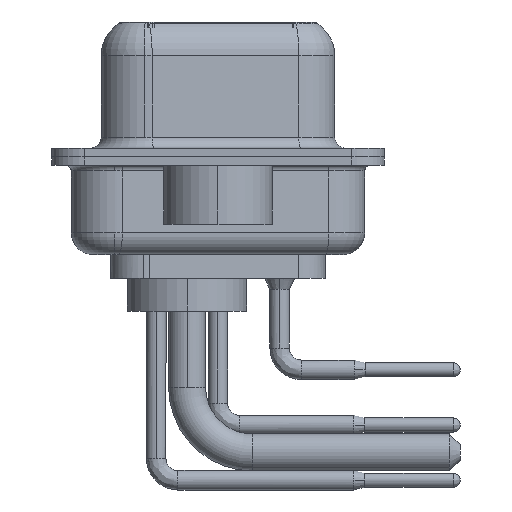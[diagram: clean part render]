
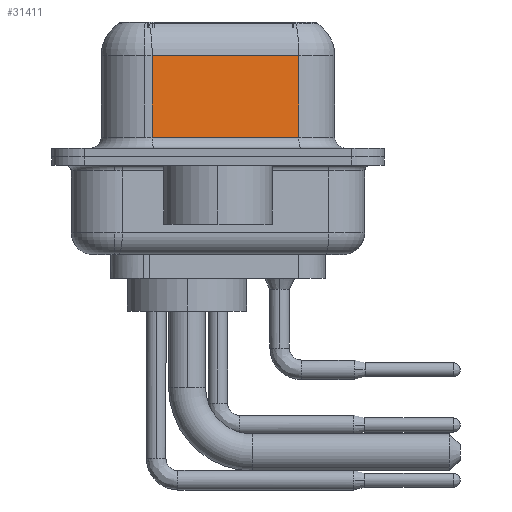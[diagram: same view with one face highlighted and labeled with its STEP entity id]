
A CAD part, left-side view. The second image highlights one B-rep face of the part: STEP entity #31411.
In plain terms, the highlighted planar face has unit normal (-0.985, -0.174, 0).
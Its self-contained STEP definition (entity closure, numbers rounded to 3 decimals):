
#448 = DIRECTION ( 'NONE',  ( 0.174, -0.985, 0. ) ) ;
#1544 = PLANE ( 'NONE',  #31819 ) ;
#2123 = EDGE_LOOP ( 'NONE', ( #21889, #3475, #9913, #14972 ) ) ;
#2804 = LINE ( 'NONE', #12839, #31920 ) ;
#3475 = ORIENTED_EDGE ( 'NONE', *, *, #16278, .T. ) ;
#3918 = DIRECTION ( 'NONE',  ( -0.174, 0.985, 0. ) ) ;
#3994 = EDGE_CURVE ( 'NONE', #17035, #30878, #7705, .T. ) ;
#4028 = DIRECTION ( 'NONE',  ( 0.985, 0.174, 0. ) ) ;
#5086 = CARTESIAN_POINT ( 'NONE',  ( 5.621, -3.722, 6.4 ) ) ;
#5248 = EDGE_CURVE ( 'NONE', #15161, #30878, #13133, .T. ) ;
#6377 = CARTESIAN_POINT ( 'NONE',  ( 5.621, -3.722, 0.9 ) ) ;
#7705 = LINE ( 'NONE', #5086, #16995 ) ;
#9243 = VECTOR ( 'NONE', #3918, 1000. ) ;
#9913 = ORIENTED_EDGE ( 'NONE', *, *, #10064, .T. ) ;
#10064 = EDGE_CURVE ( 'NONE', #23374, #15161, #2804, .T. ) ;
#10382 = DIRECTION ( 'NONE',  ( 0., 0., -1. ) ) ;
#12547 = CARTESIAN_POINT ( 'NONE',  ( 4.43, 3.028, 4.65 ) ) ;
#12839 = CARTESIAN_POINT ( 'NONE',  ( 4.43, 3.028, 6.4 ) ) ;
#13133 = LINE ( 'NONE', #32398, #14982 ) ;
#14060 = DIRECTION ( 'NONE',  ( -0.174, 0.985, 0. ) ) ;
#14972 = ORIENTED_EDGE ( 'NONE', *, *, #5248, .T. ) ;
#14982 = VECTOR ( 'NONE', #448, 1000. ) ;
#15161 = VERTEX_POINT ( 'NONE', #19263 ) ;
#16278 = EDGE_CURVE ( 'NONE', #17035, #23374, #31018, .T. ) ;
#16995 = VECTOR ( 'NONE', #25635, 1000. ) ;
#17035 = VERTEX_POINT ( 'NONE', #27219 ) ;
#19263 = CARTESIAN_POINT ( 'NONE',  ( 4.43, 3.028, 0.9 ) ) ;
#21143 = CARTESIAN_POINT ( 'NONE',  ( 5.621, -3.722, 6.4 ) ) ;
#21624 = FACE_OUTER_BOUND ( 'NONE', #2123, .T. ) ;
#21889 = ORIENTED_EDGE ( 'NONE', *, *, #3994, .F. ) ;
#23374 = VERTEX_POINT ( 'NONE', #12547 ) ;
#25635 = DIRECTION ( 'NONE',  ( 0., 0., -1. ) ) ;
#27219 = CARTESIAN_POINT ( 'NONE',  ( 5.621, -3.722, 4.65 ) ) ;
#30851 = CARTESIAN_POINT ( 'NONE',  ( 5.621, -3.722, 4.65 ) ) ;
#30878 = VERTEX_POINT ( 'NONE', #6377 ) ;
#31018 = LINE ( 'NONE', #30851, #9243 ) ;
#31411 = ADVANCED_FACE ( 'NONE', ( #21624 ), #1544, .F. ) ;
#31819 = AXIS2_PLACEMENT_3D ( 'NONE', #21143, #4028, #14060 ) ;
#31920 = VECTOR ( 'NONE', #10382, 1000. ) ;
#32398 = CARTESIAN_POINT ( 'NONE',  ( 5.621, -3.722, 0.9 ) ) ;
